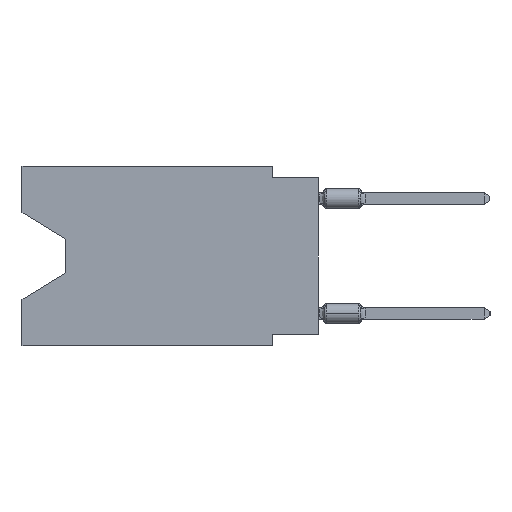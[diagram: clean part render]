
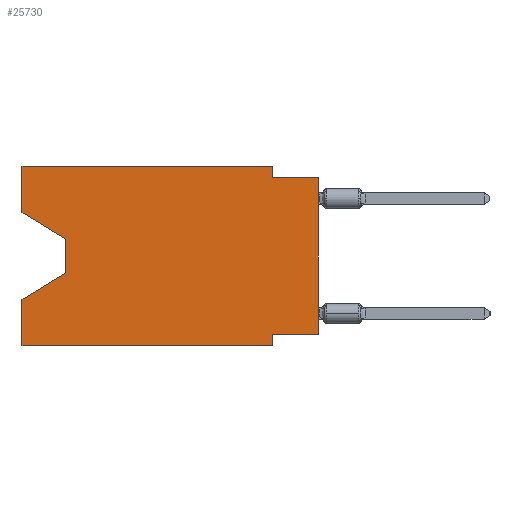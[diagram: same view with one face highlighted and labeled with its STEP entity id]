
A CAD part, left-side view. The second image highlights one B-rep face of the part: STEP entity #25730.
In plain terms, the highlighted planar face has unit normal (-1, 0, 0).
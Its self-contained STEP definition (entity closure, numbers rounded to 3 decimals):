
#920 = CARTESIAN_POINT ( 'NONE',  ( 0., 2.54, -9.906 ) ) ;
#969 = LINE ( 'NONE', #37525, #38713 ) ;
#1020 = VERTEX_POINT ( 'NONE', #54894 ) ;
#1177 = EDGE_CURVE ( 'NONE', #5335, #40867, #47092, .T. ) ;
#1591 = DIRECTION ( 'NONE',  ( 0., 0., -1. ) ) ;
#2180 = CARTESIAN_POINT ( 'NONE',  ( 0., 13.97, -5.893 ) ) ;
#2291 = VERTEX_POINT ( 'NONE', #43107 ) ;
#3918 = EDGE_LOOP ( 'NONE', ( #9180, #7879, #43196, #44511, #12219, #56620, #50937, #46777, #52484, #25254, #30127, #24376 ) ) ;
#4688 = VERTEX_POINT ( 'NONE', #6597 ) ;
#4692 = DIRECTION ( 'NONE',  ( 0., 0., -1. ) ) ;
#5335 = VERTEX_POINT ( 'NONE', #30465 ) ;
#6042 = EDGE_CURVE ( 'NONE', #12379, #2291, #969, .T. ) ;
#6443 = DIRECTION ( 'NONE',  ( 0., -1., 0. ) ) ;
#6597 = CARTESIAN_POINT ( 'NONE',  ( 0., 16.383, -9.906 ) ) ;
#6675 = DIRECTION ( 'NONE',  ( 0., 0., 1. ) ) ;
#6955 = CARTESIAN_POINT ( 'NONE',  ( 0., 0., -0.635 ) ) ;
#7879 = ORIENTED_EDGE ( 'NONE', *, *, #58787, .T. ) ;
#9036 = AXIS2_PLACEMENT_3D ( 'NONE', #17927, #40112, #26901 ) ;
#9180 = ORIENTED_EDGE ( 'NONE', *, *, #23494, .T. ) ;
#9631 = DIRECTION ( 'NONE',  ( 0., 0., -1. ) ) ;
#10066 = LINE ( 'NONE', #28318, #47810 ) ;
#11583 = DIRECTION ( 'NONE',  ( 0., -0.855, -0.519 ) ) ;
#12219 = ORIENTED_EDGE ( 'NONE', *, *, #41746, .T. ) ;
#12235 = CARTESIAN_POINT ( 'NONE',  ( 0., 0., -0.635 ) ) ;
#12379 = VERTEX_POINT ( 'NONE', #19458 ) ;
#12864 = PLANE ( 'NONE',  #9036 ) ;
#13980 = LINE ( 'NONE', #23840, #32031 ) ;
#17321 = VERTEX_POINT ( 'NONE', #19299 ) ;
#17927 = CARTESIAN_POINT ( 'NONE',  ( 0., 16.383, 0. ) ) ;
#19299 = CARTESIAN_POINT ( 'NONE',  ( 0., 0., -9.271 ) ) ;
#19458 = CARTESIAN_POINT ( 'NONE',  ( 0., 16.383, -2.546 ) ) ;
#20091 = VERTEX_POINT ( 'NONE', #20320 ) ;
#20157 = LINE ( 'NONE', #28857, #30342 ) ;
#20320 = CARTESIAN_POINT ( 'NONE',  ( 0., 2.54, 0. ) ) ;
#23458 = DIRECTION ( 'NONE',  ( 0., -1., 0. ) ) ;
#23494 = EDGE_CURVE ( 'NONE', #12379, #1020, #33759, .T. ) ;
#23840 = CARTESIAN_POINT ( 'NONE',  ( 0., 13.97, -4.013 ) ) ;
#24376 = ORIENTED_EDGE ( 'NONE', *, *, #6042, .F. ) ;
#25139 = EDGE_CURVE ( 'NONE', #2291, #20091, #52849, .T. ) ;
#25254 = ORIENTED_EDGE ( 'NONE', *, *, #28956, .F. ) ;
#25450 = VERTEX_POINT ( 'NONE', #50415 ) ;
#25628 = CARTESIAN_POINT ( 'NONE',  ( 0., 2.54, -9.271 ) ) ;
#25730 = ADVANCED_FACE ( 'NONE', ( #45172 ), #12864, .F. ) ;
#26402 = VECTOR ( 'NONE', #9631, 1000. ) ;
#26901 = DIRECTION ( 'NONE',  ( 0., 0., -1. ) ) ;
#28186 = EDGE_CURVE ( 'NONE', #39509, #25450, #32985, .T. ) ;
#28242 = LINE ( 'NONE', #33040, #29404 ) ;
#28318 = CARTESIAN_POINT ( 'NONE',  ( 0., 0., -9.271 ) ) ;
#28442 = VECTOR ( 'NONE', #6675, 1000. ) ;
#28857 = CARTESIAN_POINT ( 'NONE',  ( 0., 2.54, 0. ) ) ;
#28956 = EDGE_CURVE ( 'NONE', #20091, #5335, #20157, .T. ) ;
#29404 = VECTOR ( 'NONE', #23458, 1000. ) ;
#29800 = CARTESIAN_POINT ( 'NONE',  ( 0., 13.97, -5.893 ) ) ;
#30127 = ORIENTED_EDGE ( 'NONE', *, *, #25139, .F. ) ;
#30342 = VECTOR ( 'NONE', #1591, 1000. ) ;
#30465 = CARTESIAN_POINT ( 'NONE',  ( 0., 2.54, -0.635 ) ) ;
#30956 = VECTOR ( 'NONE', #11583, 1000. ) ;
#32031 = VECTOR ( 'NONE', #4692, 1000. ) ;
#32985 = LINE ( 'NONE', #920, #26402 ) ;
#33040 = CARTESIAN_POINT ( 'NONE',  ( 0., 16.383, -9.906 ) ) ;
#33759 = LINE ( 'NONE', #57395, #30956 ) ;
#34008 = DIRECTION ( 'NONE',  ( 0., 1., 0. ) ) ;
#34246 = DIRECTION ( 'NONE',  ( 0., 0.855, -0.519 ) ) ;
#34445 = EDGE_CURVE ( 'NONE', #17321, #40867, #39072, .T. ) ;
#37525 = CARTESIAN_POINT ( 'NONE',  ( 0., 16.383, 0. ) ) ;
#37733 = VECTOR ( 'NONE', #34246, 1000. ) ;
#38142 = LINE ( 'NONE', #2180, #37733 ) ;
#38565 = EDGE_CURVE ( 'NONE', #53401, #48415, #38142, .T. ) ;
#38713 = VECTOR ( 'NONE', #55799, 1000. ) ;
#39072 = LINE ( 'NONE', #51963, #58446 ) ;
#39509 = VERTEX_POINT ( 'NONE', #25628 ) ;
#40112 = DIRECTION ( 'NONE',  ( 1., 0., 0. ) ) ;
#40867 = VERTEX_POINT ( 'NONE', #12235 ) ;
#41746 = EDGE_CURVE ( 'NONE', #4688, #25450, #28242, .T. ) ;
#41950 = EDGE_CURVE ( 'NONE', #4688, #48415, #52198, .T. ) ;
#43107 = CARTESIAN_POINT ( 'NONE',  ( 0., 16.383, 0. ) ) ;
#43196 = ORIENTED_EDGE ( 'NONE', *, *, #38565, .T. ) ;
#43202 = VECTOR ( 'NONE', #47397, 1000. ) ;
#44511 = ORIENTED_EDGE ( 'NONE', *, *, #41950, .F. ) ;
#45172 = FACE_OUTER_BOUND ( 'NONE', #3918, .T. ) ;
#46515 = EDGE_CURVE ( 'NONE', #17321, #39509, #10066, .T. ) ;
#46777 = ORIENTED_EDGE ( 'NONE', *, *, #34445, .T. ) ;
#47092 = LINE ( 'NONE', #6955, #43202 ) ;
#47397 = DIRECTION ( 'NONE',  ( 0., -1., 0. ) ) ;
#47411 = CARTESIAN_POINT ( 'NONE',  ( 0., 16.383, 0. ) ) ;
#47810 = VECTOR ( 'NONE', #34008, 1000. ) ;
#48415 = VERTEX_POINT ( 'NONE', #48887 ) ;
#48887 = CARTESIAN_POINT ( 'NONE',  ( 0., 16.383, -7.36 ) ) ;
#50415 = CARTESIAN_POINT ( 'NONE',  ( 0., 2.54, -9.906 ) ) ;
#50937 = ORIENTED_EDGE ( 'NONE', *, *, #46515, .F. ) ;
#51963 = CARTESIAN_POINT ( 'NONE',  ( 0., 0., 0. ) ) ;
#52198 = LINE ( 'NONE', #47411, #28442 ) ;
#52484 = ORIENTED_EDGE ( 'NONE', *, *, #1177, .F. ) ;
#52849 = LINE ( 'NONE', #57045, #53910 ) ;
#53401 = VERTEX_POINT ( 'NONE', #29800 ) ;
#53910 = VECTOR ( 'NONE', #6443, 1000. ) ;
#54894 = CARTESIAN_POINT ( 'NONE',  ( 0., 13.97, -4.013 ) ) ;
#55799 = DIRECTION ( 'NONE',  ( 0., 0., 1. ) ) ;
#56620 = ORIENTED_EDGE ( 'NONE', *, *, #28186, .F. ) ;
#57045 = CARTESIAN_POINT ( 'NONE',  ( 0., 16.383, 0. ) ) ;
#57395 = CARTESIAN_POINT ( 'NONE',  ( 0., 16.383, -2.546 ) ) ;
#57629 = DIRECTION ( 'NONE',  ( 0., 0., 1. ) ) ;
#58446 = VECTOR ( 'NONE', #57629, 1000. ) ;
#58787 = EDGE_CURVE ( 'NONE', #1020, #53401, #13980, .T. ) ;
